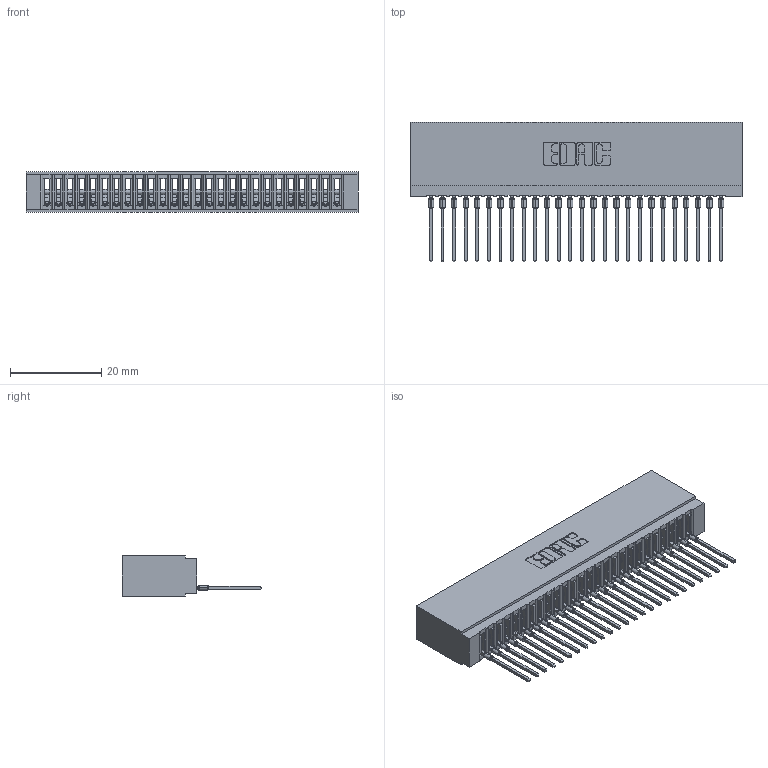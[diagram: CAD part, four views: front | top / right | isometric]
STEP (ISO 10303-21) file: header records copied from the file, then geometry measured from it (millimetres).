
FILE_DESCRIPTION (( 'STEP AP203' ), '1' );
FILE_NAME ('745-026-545-101.STEP', '2026-02-25T17:14:03', ( '' ), ( '' ), 'SwSTEP 2.0', 'SolidWorks 2023', '' );
FILE_SCHEMA (( 'CONFIG_CONTROL_DESIGN' ));
Length unit declared in the file: millimetre
Products named in the file (3): 745 Part_Insulator Option - 01; 745-292-001_545; 745-026-545-101
Assembly tree (27 placements, depth 2):
  745-026-545-101
    745 Part_Insulator Option - 01
    745-292-001_545  x26
Bounding box: 72.64 x 30.62 x 8.89 mm (x, y, z)
Volume: 6475.9 mm3; surface area: 12134.6 mm2
Topology: 27 solids, 27 shells, 3007 faces, 8266 edges, 5216 vertices
Faces by surface type: plane 1797, cylinder 534, bspline 520, torus 156
Entity records: 45124 total; most frequent: CARTESIAN_POINT 8453, ORIENTED_EDGE 7882, DIRECTION 6847, EDGE_CURVE 3941, VECTOR 3603, LINE 3603, VERTEX_POINT 2516, AXIS2_PLACEMENT_3D 1622
